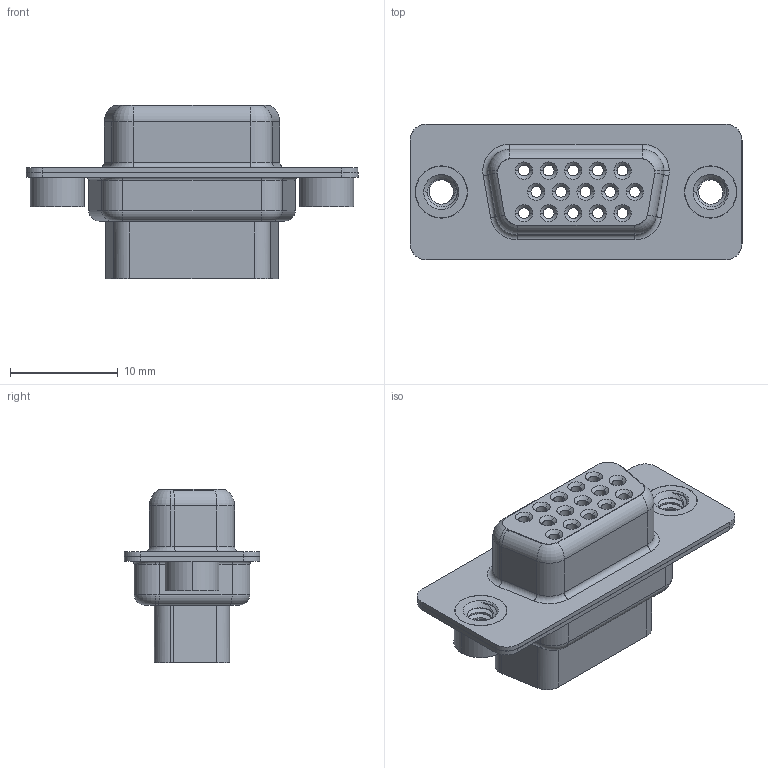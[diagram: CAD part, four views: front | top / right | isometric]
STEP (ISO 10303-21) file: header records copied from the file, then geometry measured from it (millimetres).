
FILE_DESCRIPTION (( 'STEP AP203' ), '1' );
FILE_NAME ('638-015-010-242.STEP', '2020-07-18T16:32:42', ( '' ), ( '' ), 'SwSTEP 2.0', 'SolidWorks 2020', '' );
FILE_SCHEMA (( 'CONFIG_CONTROL_DESIGN' ));
Length unit declared in the file: millimetre
Products named in the file (5): 638 Housing_15 Contacts HP; 638-015-010-242; 638 Shell Rear_15 Contacts; 638 Shell Front_15 Contacts; 638 4-40 Threaded Rivet
Assembly tree (5 placements, depth 2):
  638-015-010-242
    638 Housing_15 Contacts HP
    638 Shell Front_15 Contacts
    638 Shell Rear_15 Contacts
    638 4-40 Threaded Rivet  x2
Bounding box: 30.81 x 12.6 x 16.1 mm (x, y, z)
Volume: 1711.6 mm3; surface area: 4550.4 mm2
Topology: 5 solids, 5 shells, 474 faces, 1105 edges, 697 vertices
Faces by surface type: cylinder 257, plane 112, torus 57, cone 42, bspline 6
Entity records: 14781 total; most frequent: CARTESIAN_POINT 3779, DIRECTION 2388, ORIENTED_EDGE 2048, EDGE_CURVE 1024, AXIS2_PLACEMENT_3D 995, VERTEX_POINT 645, CIRCLE 549, EDGE_LOOP 539
